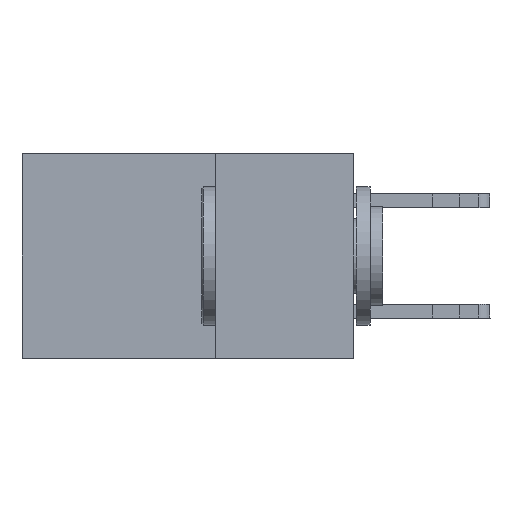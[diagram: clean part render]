
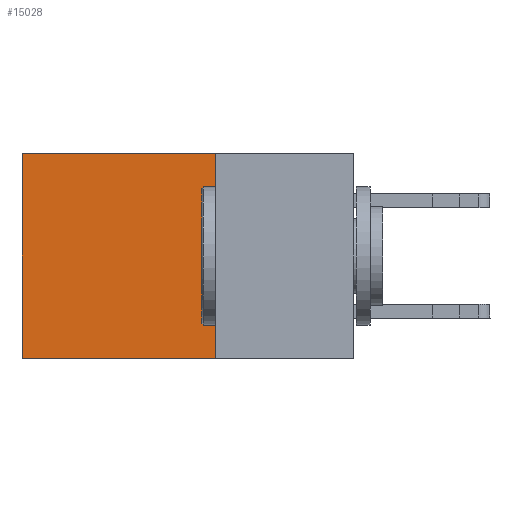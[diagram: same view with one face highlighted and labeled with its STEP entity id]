
A CAD part, left-side view. The second image highlights one B-rep face of the part: STEP entity #15028.
In plain terms, the highlighted planar face has unit normal (-1, 0, 0).
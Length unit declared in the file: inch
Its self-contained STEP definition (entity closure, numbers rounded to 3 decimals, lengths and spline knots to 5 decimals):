
#113 = LINE ( 'NONE', #15229, #22609 ) ;
#1165 = EDGE_LOOP ( 'NONE', ( #21106, #17398, #4693, #16463 ) ) ;
#1898 = DIRECTION ( 'NONE',  ( 0., 1., 0. ) ) ;
#1961 = CARTESIAN_POINT ( 'NONE',  ( 0.2875, 0.6, 0. ) ) ;
#2231 = DIRECTION ( 'NONE',  ( 0., 1., 0. ) ) ;
#3508 = LINE ( 'NONE', #10744, #21773 ) ;
#4570 = FACE_OUTER_BOUND ( 'NONE', #1165, .T. ) ;
#4693 = ORIENTED_EDGE ( 'NONE', *, *, #7331, .F. ) ;
#5536 = DIRECTION ( 'NONE',  ( 0., 0., -1. ) ) ;
#6221 = VECTOR ( 'NONE', #2231, 39.37008 ) ;
#6410 = VERTEX_POINT ( 'NONE', #19969 ) ;
#7331 = EDGE_CURVE ( 'NONE', #10151, #23033, #113, .T. ) ;
#7569 = CARTESIAN_POINT ( 'NONE',  ( 0.2875, 0.25, -0.37 ) ) ;
#7614 = EDGE_CURVE ( 'NONE', #23033, #6410, #3508, .T. ) ;
#8544 = PLANE ( 'NONE',  #22794 ) ;
#10079 = DIRECTION ( 'NONE',  ( 0., 0., -1. ) ) ;
#10151 = VERTEX_POINT ( 'NONE', #22511 ) ;
#10305 = DIRECTION ( 'NONE',  ( 1., 0., 0. ) ) ;
#10744 = CARTESIAN_POINT ( 'NONE',  ( 0.2875, 0.25, -0.37 ) ) ;
#11022 = EDGE_CURVE ( 'NONE', #13206, #6410, #14128, .T. ) ;
#11298 = CARTESIAN_POINT ( 'NONE',  ( 0.2875, 0.6, 0. ) ) ;
#12866 = CARTESIAN_POINT ( 'NONE',  ( 0.2875, 0.25, 0. ) ) ;
#13206 = VERTEX_POINT ( 'NONE', #11298 ) ;
#13574 = VECTOR ( 'NONE', #5536, 39.37008 ) ;
#14128 = LINE ( 'NONE', #1961, #13574 ) ;
#15028 = ADVANCED_FACE ( 'NONE', ( #4570 ), #8544, .F. ) ;
#15037 = LINE ( 'NONE', #12866, #6221 ) ;
#15229 = CARTESIAN_POINT ( 'NONE',  ( 0.2875, 0.25, 0. ) ) ;
#16463 = ORIENTED_EDGE ( 'NONE', *, *, #21181, .T. ) ;
#17398 = ORIENTED_EDGE ( 'NONE', *, *, #7614, .F. ) ;
#19969 = CARTESIAN_POINT ( 'NONE',  ( 0.2875, 0.6, -0.37 ) ) ;
#20908 = CARTESIAN_POINT ( 'NONE',  ( 0.2875, 0.25, 0. ) ) ;
#21106 = ORIENTED_EDGE ( 'NONE', *, *, #11022, .T. ) ;
#21181 = EDGE_CURVE ( 'NONE', #10151, #13206, #15037, .T. ) ;
#21773 = VECTOR ( 'NONE', #1898, 39.37008 ) ;
#22511 = CARTESIAN_POINT ( 'NONE',  ( 0.2875, 0.25, 0. ) ) ;
#22609 = VECTOR ( 'NONE', #10079, 39.37008 ) ;
#22658 = DIRECTION ( 'NONE',  ( 0., 0., -1. ) ) ;
#22794 = AXIS2_PLACEMENT_3D ( 'NONE', #20908, #10305, #22658 ) ;
#23033 = VERTEX_POINT ( 'NONE', #7569 ) ;
